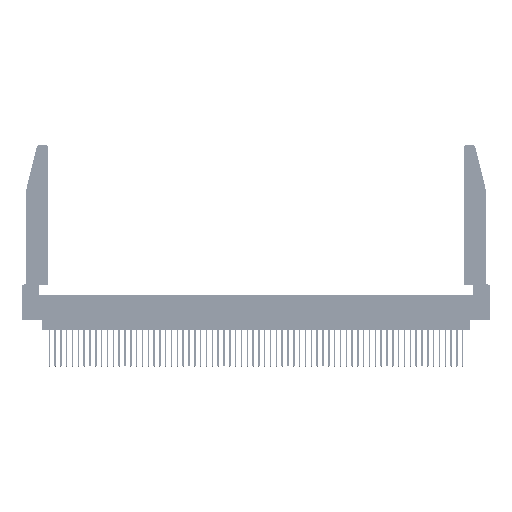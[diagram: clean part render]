
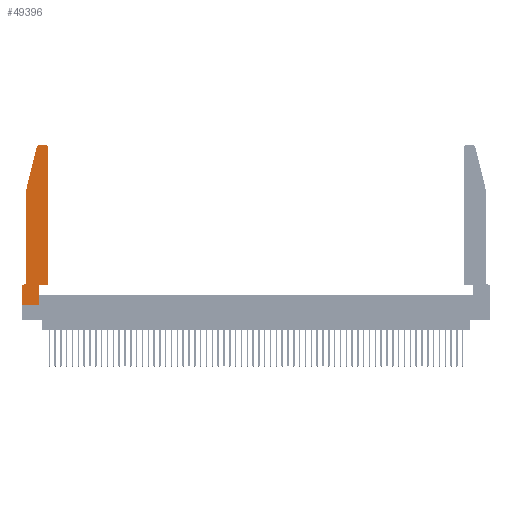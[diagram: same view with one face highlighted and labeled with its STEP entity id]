
A CAD part, top view. The second image highlights one B-rep face of the part: STEP entity #49396.
In plain terms, the highlighted planar face has unit normal (0, 0, 1).
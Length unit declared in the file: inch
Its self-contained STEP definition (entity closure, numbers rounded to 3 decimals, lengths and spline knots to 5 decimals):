
#414 = CARTESIAN_POINT ( 'NONE',  ( 0., 0., 0.37 ) ) ;
#691 = VECTOR ( 'NONE', #4818, 39.37008 ) ;
#848 = CARTESIAN_POINT ( 'NONE',  ( 0., 0., 0.37 ) ) ;
#984 = CARTESIAN_POINT ( 'NONE',  ( 0.4505, 0.35, 0.37 ) ) ;
#2821 = EDGE_CURVE ( 'NONE', #18953, #23900, #36588, .T. ) ;
#4284 = VERTEX_POINT ( 'NONE', #8918 ) ;
#4818 = DIRECTION ( 'NONE',  ( 1., 0., 0. ) ) ;
#6727 = FACE_OUTER_BOUND ( 'NONE', #45540, .T. ) ;
#8031 = DIRECTION ( 'NONE',  ( 0., 0., 1. ) ) ;
#8908 = ORIENTED_EDGE ( 'NONE', *, *, #39886, .T. ) ;
#8918 = CARTESIAN_POINT ( 'NONE',  ( 0.2865, 0.35, 0.37 ) ) ;
#10341 = CARTESIAN_POINT ( 'NONE',  ( 0.284, 2.72, 0.37 ) ) ;
#10431 = CARTESIAN_POINT ( 'NONE',  ( 0., 0., 0.37 ) ) ;
#10817 = VERTEX_POINT ( 'NONE', #848 ) ;
#13057 = ORIENTED_EDGE ( 'NONE', *, *, #16076, .T. ) ;
#13276 = DIRECTION ( 'NONE',  ( 1., 0., 0. ) ) ;
#14362 = CIRCLE ( 'NONE', #53228, 0.03 ) ;
#15591 = VERTEX_POINT ( 'NONE', #42248 ) ;
#16076 = EDGE_CURVE ( 'NONE', #4284, #53338, #36202, .T. ) ;
#16335 = CIRCLE ( 'NONE', #40704, 0.03 ) ;
#17038 = AXIS2_PLACEMENT_3D ( 'NONE', #46069, #54437, #32292 ) ;
#17767 = EDGE_CURVE ( 'NONE', #10817, #44190, #41559, .T. ) ;
#18953 = VERTEX_POINT ( 'NONE', #36079 ) ;
#19250 = LINE ( 'NONE', #46159, #40739 ) ;
#19939 = ORIENTED_EDGE ( 'NONE', *, *, #2821, .T. ) ;
#21397 = VERTEX_POINT ( 'NONE', #48793 ) ;
#21739 = ORIENTED_EDGE ( 'NONE', *, *, #40979, .T. ) ;
#23048 = LINE ( 'NONE', #54427, #54270 ) ;
#23900 = VERTEX_POINT ( 'NONE', #43302 ) ;
#26375 = LINE ( 'NONE', #50655, #49991 ) ;
#26872 = VECTOR ( 'NONE', #50740, 39.37008 ) ;
#27876 = CARTESIAN_POINT ( 'NONE',  ( 0.2865, 0., 0.37 ) ) ;
#28134 = ORIENTED_EDGE ( 'NONE', *, *, #56054, .T. ) ;
#30163 = AXIS2_PLACEMENT_3D ( 'NONE', #39382, #8031, #56673 ) ;
#30584 = ORIENTED_EDGE ( 'NONE', *, *, #46465, .T. ) ;
#31099 = ORIENTED_EDGE ( 'NONE', *, *, #43733, .T. ) ;
#32110 = CARTESIAN_POINT ( 'NONE',  ( 0.2605, 2.75, 0.37 ) ) ;
#32173 = VERTEX_POINT ( 'NONE', #43742 ) ;
#32292 = DIRECTION ( 'NONE',  ( -1., 0., 0. ) ) ;
#32409 = EDGE_CURVE ( 'NONE', #21397, #10817, #33181, .T. ) ;
#33105 = LINE ( 'NONE', #32110, #26872 ) ;
#33181 = LINE ( 'NONE', #10431, #40787 ) ;
#33189 = EDGE_CURVE ( 'NONE', #44190, #4284, #19250, .T. ) ;
#33329 = CARTESIAN_POINT ( 'NONE',  ( 0.0055, 0.35, 0.37 ) ) ;
#34021 = VECTOR ( 'NONE', #44703, 39.37008 ) ;
#34092 = VECTOR ( 'NONE', #36356, 39.37008 ) ;
#35518 = DIRECTION ( 'NONE',  ( 0., 0., 1. ) ) ;
#36079 = CARTESIAN_POINT ( 'NONE',  ( 0.25487, 2.72718, 0.37 ) ) ;
#36202 = LINE ( 'NONE', #984, #34092 ) ;
#36356 = DIRECTION ( 'NONE',  ( 1., 0., 0. ) ) ;
#36588 = LINE ( 'NONE', #50731, #45623 ) ;
#37230 = DIRECTION ( 'NONE',  ( 0., 1., 0. ) ) ;
#37503 = DIRECTION ( 'NONE',  ( -0.239, -0.971, 0. ) ) ;
#37504 = EDGE_CURVE ( 'NONE', #23900, #57348, #54881, .T. ) ;
#37779 = CARTESIAN_POINT ( 'NONE',  ( 0.4505, 0.35, 0.37 ) ) ;
#38957 = DIRECTION ( 'NONE',  ( -1., 0., 0. ) ) ;
#39007 = PLANE ( 'NONE',  #30163 ) ;
#39382 = CARTESIAN_POINT ( 'NONE',  ( 0., 0.35, 0.37 ) ) ;
#39886 = EDGE_CURVE ( 'NONE', #52568, #15591, #33105, .T. ) ;
#40447 = CIRCLE ( 'NONE', #17038, 0.07 ) ;
#40704 = AXIS2_PLACEMENT_3D ( 'NONE', #10341, #41475, #54321 ) ;
#40739 = VECTOR ( 'NONE', #50056, 39.37008 ) ;
#40787 = VECTOR ( 'NONE', #40788, 39.37008 ) ;
#40788 = DIRECTION ( 'NONE',  ( 0., -1., 0. ) ) ;
#40979 = EDGE_CURVE ( 'NONE', #15591, #18953, #16335, .T. ) ;
#41115 = VERTEX_POINT ( 'NONE', #33329 ) ;
#41475 = DIRECTION ( 'NONE',  ( 0., 0., 1. ) ) ;
#41559 = LINE ( 'NONE', #414, #691 ) ;
#42248 = CARTESIAN_POINT ( 'NONE',  ( 0.284, 2.75, 0.37 ) ) ;
#42264 = ORIENTED_EDGE ( 'NONE', *, *, #37504, .T. ) ;
#43302 = CARTESIAN_POINT ( 'NONE',  ( 0.0755, 2., 0.37 ) ) ;
#43733 = EDGE_CURVE ( 'NONE', #53338, #32173, #26375, .T. ) ;
#43742 = CARTESIAN_POINT ( 'NONE',  ( 0.4505, 2.72, 0.37 ) ) ;
#44190 = VERTEX_POINT ( 'NONE', #27876 ) ;
#44703 = DIRECTION ( 'NONE',  ( 0., -1., 0. ) ) ;
#45540 = EDGE_LOOP ( 'NONE', ( #8908, #21739, #19939, #42264, #28134, #30584, #54781, #52007, #57127, #13057, #31099, #52451 ) ) ;
#45623 = VECTOR ( 'NONE', #37503, 39.37008 ) ;
#45924 = CARTESIAN_POINT ( 'NONE',  ( 0.0755, 0.42, 0.37 ) ) ;
#46069 = CARTESIAN_POINT ( 'NONE',  ( 0.0055, 0.42, 0.37 ) ) ;
#46159 = CARTESIAN_POINT ( 'NONE',  ( 0.2865, 0.35, 0.37 ) ) ;
#46465 = EDGE_CURVE ( 'NONE', #41115, #21397, #23048, .T. ) ;
#48793 = CARTESIAN_POINT ( 'NONE',  ( 0., 0.35, 0.37 ) ) ;
#49134 = CARTESIAN_POINT ( 'NONE',  ( 0.4205, 2.75, 0.37 ) ) ;
#49396 = ADVANCED_FACE ( 'NONE', ( #6727 ), #39007, .T. ) ;
#49503 = EDGE_CURVE ( 'NONE', #32173, #52568, #14362, .T. ) ;
#49991 = VECTOR ( 'NONE', #37230, 39.37008 ) ;
#50056 = DIRECTION ( 'NONE',  ( 0., 1., 0. ) ) ;
#50655 = CARTESIAN_POINT ( 'NONE',  ( 0.4505, 0.35, 0.37 ) ) ;
#50731 = CARTESIAN_POINT ( 'NONE',  ( 0.0755, 2., 0.37 ) ) ;
#50740 = DIRECTION ( 'NONE',  ( -1., 0., 0. ) ) ;
#52007 = ORIENTED_EDGE ( 'NONE', *, *, #17767, .T. ) ;
#52451 = ORIENTED_EDGE ( 'NONE', *, *, #49503, .T. ) ;
#52568 = VERTEX_POINT ( 'NONE', #49134 ) ;
#53228 = AXIS2_PLACEMENT_3D ( 'NONE', #53934, #35518, #13276 ) ;
#53338 = VERTEX_POINT ( 'NONE', #37779 ) ;
#53475 = CARTESIAN_POINT ( 'NONE',  ( 0.0755, 2., 0.37 ) ) ;
#53934 = CARTESIAN_POINT ( 'NONE',  ( 0.4205, 2.72, 0.37 ) ) ;
#54270 = VECTOR ( 'NONE', #38957, 39.37008 ) ;
#54321 = DIRECTION ( 'NONE',  ( 1., 0., 0. ) ) ;
#54427 = CARTESIAN_POINT ( 'NONE',  ( 0.0755, 0.35, 0.37 ) ) ;
#54437 = DIRECTION ( 'NONE',  ( 0., 0., -1. ) ) ;
#54781 = ORIENTED_EDGE ( 'NONE', *, *, #32409, .T. ) ;
#54881 = LINE ( 'NONE', #53475, #34021 ) ;
#56054 = EDGE_CURVE ( 'NONE', #57348, #41115, #40447, .T. ) ;
#56673 = DIRECTION ( 'NONE',  ( 1., 0., 0. ) ) ;
#57127 = ORIENTED_EDGE ( 'NONE', *, *, #33189, .T. ) ;
#57348 = VERTEX_POINT ( 'NONE', #45924 ) ;
